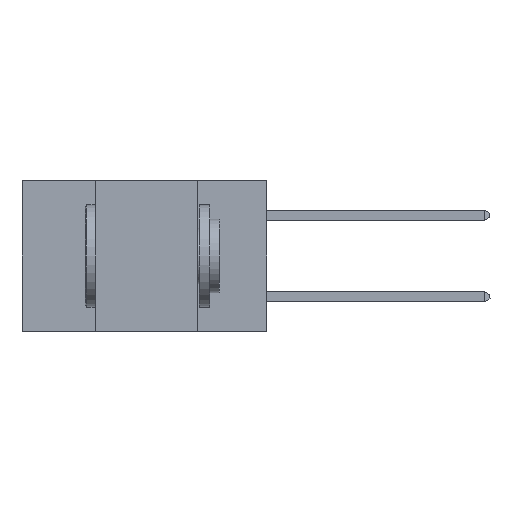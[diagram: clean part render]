
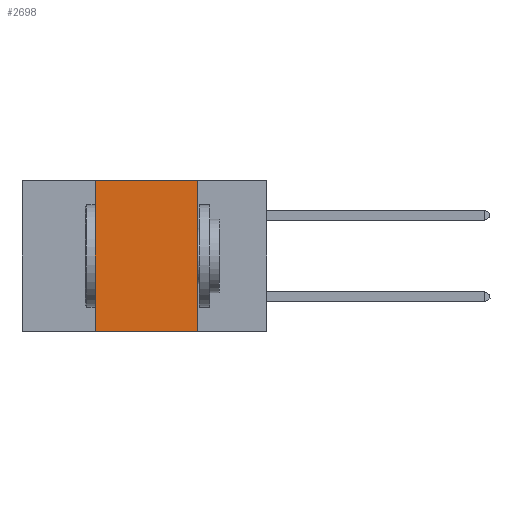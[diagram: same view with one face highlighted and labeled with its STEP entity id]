
A CAD part, left-side view. The second image highlights one B-rep face of the part: STEP entity #2698.
In plain terms, the highlighted planar face has unit normal (-1, 0, 0).
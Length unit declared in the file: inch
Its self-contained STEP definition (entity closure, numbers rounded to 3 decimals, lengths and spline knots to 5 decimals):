
#209 = VECTOR ( 'NONE', #600, 39.37008 ) ;
#235 = AXIS2_PLACEMENT_3D ( 'NONE', #1823, #7406, #401 ) ;
#367 = CARTESIAN_POINT ( 'NONE',  ( 0., 0.6, -0.37 ) ) ;
#401 = DIRECTION ( 'NONE',  ( 0., 0., -1. ) ) ;
#600 = DIRECTION ( 'NONE',  ( 0., 0., 1. ) ) ;
#729 = CARTESIAN_POINT ( 'NONE',  ( 0., 0.42, 0. ) ) ;
#980 = PLANE ( 'NONE',  #235 ) ;
#1565 = FACE_OUTER_BOUND ( 'NONE', #4485, .T. ) ;
#1776 = EDGE_CURVE ( 'NONE', #7161, #2753, #5048, .T. ) ;
#1823 = CARTESIAN_POINT ( 'NONE',  ( 0., 0.6, 0. ) ) ;
#1858 = CARTESIAN_POINT ( 'NONE',  ( 0., 0.17, -0.37 ) ) ;
#2299 = DIRECTION ( 'NONE',  ( 0., 0., -1. ) ) ;
#2305 = ORIENTED_EDGE ( 'NONE', *, *, #5734, .F. ) ;
#2698 = ADVANCED_FACE ( 'NONE', ( #1565 ), #980, .F. ) ;
#2753 = VERTEX_POINT ( 'NONE', #1858 ) ;
#3092 = EDGE_CURVE ( 'NONE', #10101, #7161, #5513, .T. ) ;
#4047 = CARTESIAN_POINT ( 'NONE',  ( 0., 0.6, 0. ) ) ;
#4485 = EDGE_LOOP ( 'NONE', ( #9627, #5891, #2305, #10013 ) ) ;
#4751 = DIRECTION ( 'NONE',  ( 0., -1., 0. ) ) ;
#4811 = DIRECTION ( 'NONE',  ( 0., -1., 0. ) ) ;
#4816 = CARTESIAN_POINT ( 'NONE',  ( 0., 0.42, 0. ) ) ;
#5048 = LINE ( 'NONE', #8753, #8185 ) ;
#5513 = LINE ( 'NONE', #4047, #7549 ) ;
#5734 = EDGE_CURVE ( 'NONE', #10047, #10101, #6350, .T. ) ;
#5891 = ORIENTED_EDGE ( 'NONE', *, *, #3092, .F. ) ;
#5927 = EDGE_CURVE ( 'NONE', #10047, #2753, #5962, .T. ) ;
#5962 = LINE ( 'NONE', #367, #7104 ) ;
#6350 = LINE ( 'NONE', #729, #209 ) ;
#6649 = CARTESIAN_POINT ( 'NONE',  ( 0., 0.42, -0.37 ) ) ;
#7005 = CARTESIAN_POINT ( 'NONE',  ( 0., 0.17, 0. ) ) ;
#7104 = VECTOR ( 'NONE', #4751, 39.37008 ) ;
#7161 = VERTEX_POINT ( 'NONE', #7005 ) ;
#7406 = DIRECTION ( 'NONE',  ( 1., 0., 0. ) ) ;
#7549 = VECTOR ( 'NONE', #4811, 39.37008 ) ;
#8185 = VECTOR ( 'NONE', #2299, 39.37008 ) ;
#8753 = CARTESIAN_POINT ( 'NONE',  ( 0., 0.17, 0. ) ) ;
#9627 = ORIENTED_EDGE ( 'NONE', *, *, #1776, .F. ) ;
#10013 = ORIENTED_EDGE ( 'NONE', *, *, #5927, .T. ) ;
#10047 = VERTEX_POINT ( 'NONE', #6649 ) ;
#10101 = VERTEX_POINT ( 'NONE', #4816 ) ;
